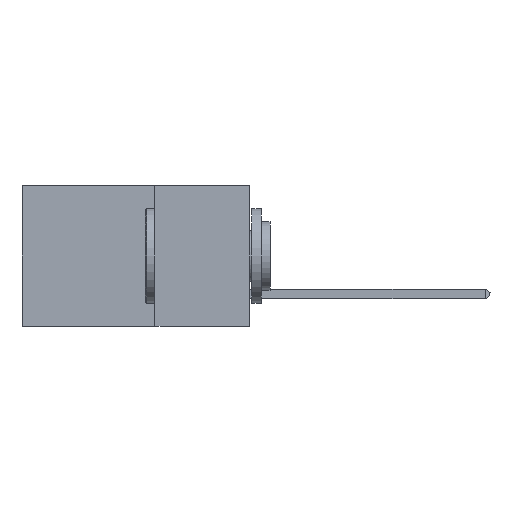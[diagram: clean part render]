
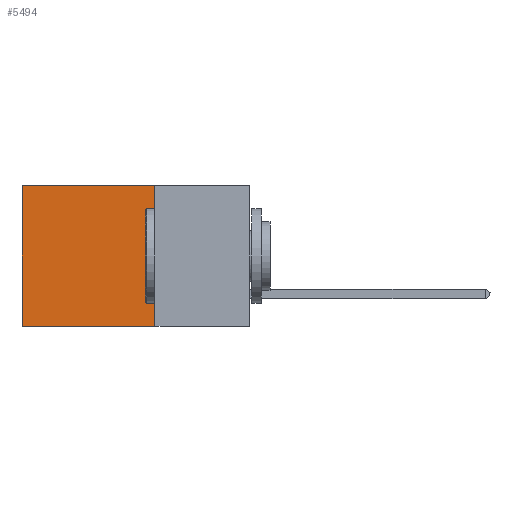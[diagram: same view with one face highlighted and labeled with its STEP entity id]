
A CAD part, left-side view. The second image highlights one B-rep face of the part: STEP entity #5494.
In plain terms, the highlighted planar face has unit normal (-1, 0, 0).
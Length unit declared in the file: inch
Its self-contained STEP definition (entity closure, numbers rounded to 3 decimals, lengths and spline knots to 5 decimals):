
#40 = EDGE_LOOP ( 'NONE', ( #7710, #8669, #20486, #20625 ) ) ;
#375 = EDGE_CURVE ( 'NONE', #18001, #19766, #5586, .T. ) ;
#544 = EDGE_CURVE ( 'NONE', #19766, #6948, #28105, .T. ) ;
#1287 = CARTESIAN_POINT ( 'NONE',  ( 0.2875, 0.6, -0.37 ) ) ;
#2461 = VECTOR ( 'NONE', #15086, 39.37008 ) ;
#5027 = AXIS2_PLACEMENT_3D ( 'NONE', #8480, #31479, #8698 ) ;
#5494 = ADVANCED_FACE ( 'NONE', ( #12753 ), #19301, .F. ) ;
#5586 = LINE ( 'NONE', #8450, #26315 ) ;
#6394 = CARTESIAN_POINT ( 'NONE',  ( 0.2875, 0.25, -0.37 ) ) ;
#6948 = VERTEX_POINT ( 'NONE', #1287 ) ;
#7710 = ORIENTED_EDGE ( 'NONE', *, *, #22141, .T. ) ;
#8450 = CARTESIAN_POINT ( 'NONE',  ( 0.2875, 0.25, 0. ) ) ;
#8480 = CARTESIAN_POINT ( 'NONE',  ( 0.2875, 0.25, 0. ) ) ;
#8669 = ORIENTED_EDGE ( 'NONE', *, *, #544, .F. ) ;
#8698 = DIRECTION ( 'NONE',  ( 0., 0., -1. ) ) ;
#12753 = FACE_OUTER_BOUND ( 'NONE', #40, .T. ) ;
#15077 = CARTESIAN_POINT ( 'NONE',  ( 0.2875, 0.6, 0. ) ) ;
#15086 = DIRECTION ( 'NONE',  ( 0., 0., -1. ) ) ;
#16096 = CARTESIAN_POINT ( 'NONE',  ( 0.2875, 0.25, 0. ) ) ;
#18001 = VERTEX_POINT ( 'NONE', #16096 ) ;
#18602 = CARTESIAN_POINT ( 'NONE',  ( 0.2875, 0.25, 0. ) ) ;
#18906 = VECTOR ( 'NONE', #32411, 39.37008 ) ;
#19301 = PLANE ( 'NONE',  #5027 ) ;
#19659 = LINE ( 'NONE', #25720, #2461 ) ;
#19766 = VERTEX_POINT ( 'NONE', #35412 ) ;
#20036 = EDGE_CURVE ( 'NONE', #18001, #22628, #34766, .T. ) ;
#20486 = ORIENTED_EDGE ( 'NONE', *, *, #375, .F. ) ;
#20625 = ORIENTED_EDGE ( 'NONE', *, *, #20036, .T. ) ;
#22141 = EDGE_CURVE ( 'NONE', #22628, #6948, #19659, .T. ) ;
#22628 = VERTEX_POINT ( 'NONE', #15077 ) ;
#23457 = DIRECTION ( 'NONE',  ( 0., 1., 0. ) ) ;
#25466 = VECTOR ( 'NONE', #23457, 39.37008 ) ;
#25720 = CARTESIAN_POINT ( 'NONE',  ( 0.2875, 0.6, 0. ) ) ;
#26315 = VECTOR ( 'NONE', #28155, 39.37008 ) ;
#28105 = LINE ( 'NONE', #6394, #25466 ) ;
#28155 = DIRECTION ( 'NONE',  ( 0., 0., -1. ) ) ;
#31479 = DIRECTION ( 'NONE',  ( 1., 0., 0. ) ) ;
#32411 = DIRECTION ( 'NONE',  ( 0., 1., 0. ) ) ;
#34766 = LINE ( 'NONE', #18602, #18906 ) ;
#35412 = CARTESIAN_POINT ( 'NONE',  ( 0.2875, 0.25, -0.37 ) ) ;
